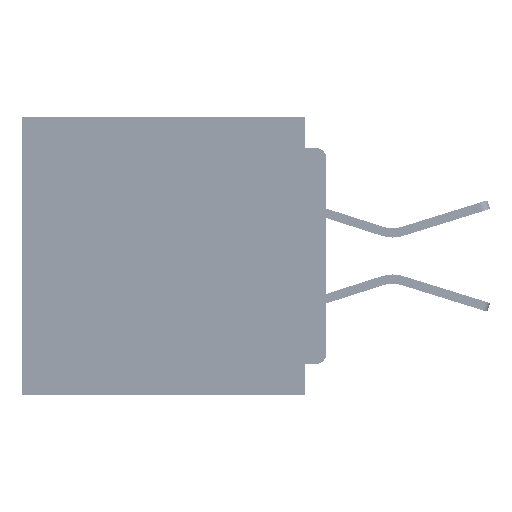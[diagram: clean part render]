
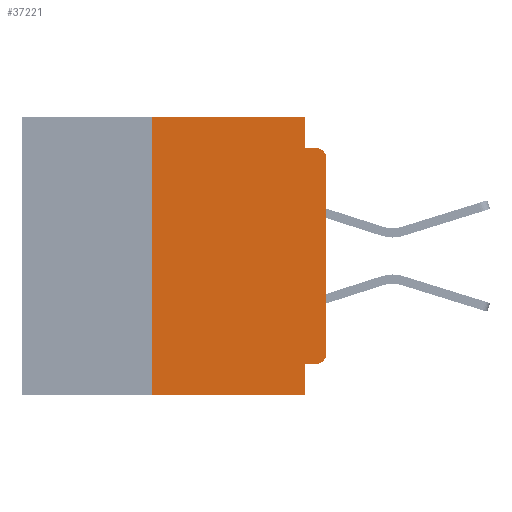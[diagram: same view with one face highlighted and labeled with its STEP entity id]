
A CAD part, left-side view. The second image highlights one B-rep face of the part: STEP entity #37221.
In plain terms, the highlighted planar face has unit normal (-1, 0, 0).
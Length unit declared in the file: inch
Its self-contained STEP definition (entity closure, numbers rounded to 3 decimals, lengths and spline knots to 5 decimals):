
#129 = ORIENTED_EDGE ( 'NONE', *, *, #37862, .F. ) ;
#2108 = VERTEX_POINT ( 'NONE', #46743 ) ;
#3139 = DIRECTION ( 'NONE',  ( 0., 0., 1. ) ) ;
#3158 = CARTESIAN_POINT ( 'NONE',  ( 0., 0., -0.045 ) ) ;
#3950 = CARTESIAN_POINT ( 'NONE',  ( 0., 0., -0.34 ) ) ;
#5666 = VECTOR ( 'NONE', #47244, 39.37008 ) ;
#5897 = CARTESIAN_POINT ( 'NONE',  ( 0., 0., -0.355 ) ) ;
#7354 = ORIENTED_EDGE ( 'NONE', *, *, #60327, .F. ) ;
#8446 = DIRECTION ( 'NONE',  ( 0., -1., 0. ) ) ;
#8626 = VERTEX_POINT ( 'NONE', #39455 ) ;
#9500 = CIRCLE ( 'NONE', #14968, 0.015 ) ;
#11223 = LINE ( 'NONE', #3158, #50873 ) ;
#11317 = LINE ( 'NONE', #58134, #63042 ) ;
#13856 = EDGE_LOOP ( 'NONE', ( #20117, #29743, #61178, #18373, #40116, #129, #65933, #27570, #7354, #15397 ) ) ;
#14566 = FACE_OUTER_BOUND ( 'NONE', #13856, .T. ) ;
#14968 = AXIS2_PLACEMENT_3D ( 'NONE', #25441, #61449, #30588 ) ;
#15135 = VECTOR ( 'NONE', #23006, 39.37008 ) ;
#15149 = DIRECTION ( 'NONE',  ( 0., -1., 0. ) ) ;
#15397 = ORIENTED_EDGE ( 'NONE', *, *, #56770, .T. ) ;
#16800 = CARTESIAN_POINT ( 'NONE',  ( 0., 0.031, 0. ) ) ;
#17708 = VERTEX_POINT ( 'NONE', #20935 ) ;
#17837 = EDGE_CURVE ( 'NONE', #20039, #2108, #56337, .T. ) ;
#18373 = ORIENTED_EDGE ( 'NONE', *, *, #37291, .F. ) ;
#19423 = CIRCLE ( 'NONE', #32344, 0.015 ) ;
#20039 = VERTEX_POINT ( 'NONE', #61693 ) ;
#20117 = ORIENTED_EDGE ( 'NONE', *, *, #45998, .T. ) ;
#20651 = PLANE ( 'NONE',  #30716 ) ;
#20935 = CARTESIAN_POINT ( 'NONE',  ( 0., 0.031, -0.355 ) ) ;
#21904 = VECTOR ( 'NONE', #42803, 39.37008 ) ;
#22152 = CARTESIAN_POINT ( 'NONE',  ( 0., 0.031, -0.045 ) ) ;
#22717 = EDGE_CURVE ( 'NONE', #64489, #50736, #19423, .T. ) ;
#22872 = EDGE_CURVE ( 'NONE', #34727, #50736, #11223, .T. ) ;
#23006 = DIRECTION ( 'NONE',  ( 0., -1., 0. ) ) ;
#25441 = CARTESIAN_POINT ( 'NONE',  ( 0., 0.015, -0.34 ) ) ;
#25531 = CARTESIAN_POINT ( 'NONE',  ( 0., 0.25, -0.4 ) ) ;
#25912 = DIRECTION ( 'NONE',  ( 1., 0., 0. ) ) ;
#27570 = ORIENTED_EDGE ( 'NONE', *, *, #62024, .F. ) ;
#28097 = CARTESIAN_POINT ( 'NONE',  ( 0., 0.015, -0.06 ) ) ;
#29378 = LINE ( 'NONE', #46124, #55165 ) ;
#29743 = ORIENTED_EDGE ( 'NONE', *, *, #22717, .T. ) ;
#30520 = LINE ( 'NONE', #61431, #42640 ) ;
#30588 = DIRECTION ( 'NONE',  ( 0., 0., -1. ) ) ;
#30716 = AXIS2_PLACEMENT_3D ( 'NONE', #56743, #25912, #61902 ) ;
#32344 = AXIS2_PLACEMENT_3D ( 'NONE', #28097, #64132, #33302 ) ;
#32498 = DIRECTION ( 'NONE',  ( 0., 0., -1. ) ) ;
#33302 = DIRECTION ( 'NONE',  ( 0., 0., -1. ) ) ;
#34394 = CARTESIAN_POINT ( 'NONE',  ( 0., 0.25, -0.4 ) ) ;
#34727 = VERTEX_POINT ( 'NONE', #22152 ) ;
#35034 = LINE ( 'NONE', #5897, #5666 ) ;
#35548 = DIRECTION ( 'NONE',  ( 0., 0., 1. ) ) ;
#35664 = LINE ( 'NONE', #16800, #21904 ) ;
#36687 = LINE ( 'NONE', #34394, #38300 ) ;
#37221 = ADVANCED_FACE ( 'NONE', ( #14566 ), #20651, .F. ) ;
#37244 = CARTESIAN_POINT ( 'NONE',  ( 0., 0.015, -0.355 ) ) ;
#37291 = EDGE_CURVE ( 'NONE', #2108, #34727, #35664, .T. ) ;
#37862 = EDGE_CURVE ( 'NONE', #58002, #20039, #36687, .T. ) ;
#38300 = VECTOR ( 'NONE', #3139, 39.37008 ) ;
#38560 = VERTEX_POINT ( 'NONE', #3950 ) ;
#39455 = CARTESIAN_POINT ( 'NONE',  ( 0., 0.031, -0.4 ) ) ;
#40116 = ORIENTED_EDGE ( 'NONE', *, *, #17837, .F. ) ;
#42640 = VECTOR ( 'NONE', #35548, 39.37008 ) ;
#42803 = DIRECTION ( 'NONE',  ( 0., 0., -1. ) ) ;
#45998 = EDGE_CURVE ( 'NONE', #38560, #64489, #30520, .T. ) ;
#46124 = CARTESIAN_POINT ( 'NONE',  ( 0., 0.437, -0.4 ) ) ;
#46743 = CARTESIAN_POINT ( 'NONE',  ( 0., 0.031, 0. ) ) ;
#47244 = DIRECTION ( 'NONE',  ( 0., 1., 0. ) ) ;
#50736 = VERTEX_POINT ( 'NONE', #58048 ) ;
#50873 = VECTOR ( 'NONE', #8446, 39.37008 ) ;
#55165 = VECTOR ( 'NONE', #15149, 39.37008 ) ;
#56337 = LINE ( 'NONE', #64013, #15135 ) ;
#56743 = CARTESIAN_POINT ( 'NONE',  ( 0., 0.437, 0. ) ) ;
#56770 = EDGE_CURVE ( 'NONE', #66159, #38560, #9500, .T. ) ;
#58002 = VERTEX_POINT ( 'NONE', #25531 ) ;
#58048 = CARTESIAN_POINT ( 'NONE',  ( 0., 0.015, -0.045 ) ) ;
#58134 = CARTESIAN_POINT ( 'NONE',  ( 0., 0.031, -0.4 ) ) ;
#60143 = EDGE_CURVE ( 'NONE', #58002, #8626, #29378, .T. ) ;
#60327 = EDGE_CURVE ( 'NONE', #66159, #17708, #35034, .T. ) ;
#61178 = ORIENTED_EDGE ( 'NONE', *, *, #22872, .F. ) ;
#61431 = CARTESIAN_POINT ( 'NONE',  ( 0., 0., 0. ) ) ;
#61449 = DIRECTION ( 'NONE',  ( -1., 0., 0. ) ) ;
#61693 = CARTESIAN_POINT ( 'NONE',  ( 0., 0.25, 0. ) ) ;
#61902 = DIRECTION ( 'NONE',  ( 0., 0., -1. ) ) ;
#62024 = EDGE_CURVE ( 'NONE', #17708, #8626, #11317, .T. ) ;
#63042 = VECTOR ( 'NONE', #32498, 39.37008 ) ;
#63496 = CARTESIAN_POINT ( 'NONE',  ( 0., 0., -0.06 ) ) ;
#64013 = CARTESIAN_POINT ( 'NONE',  ( 0., 0.437, 0. ) ) ;
#64132 = DIRECTION ( 'NONE',  ( -1., 0., 0. ) ) ;
#64489 = VERTEX_POINT ( 'NONE', #63496 ) ;
#65933 = ORIENTED_EDGE ( 'NONE', *, *, #60143, .T. ) ;
#66159 = VERTEX_POINT ( 'NONE', #37244 ) ;
